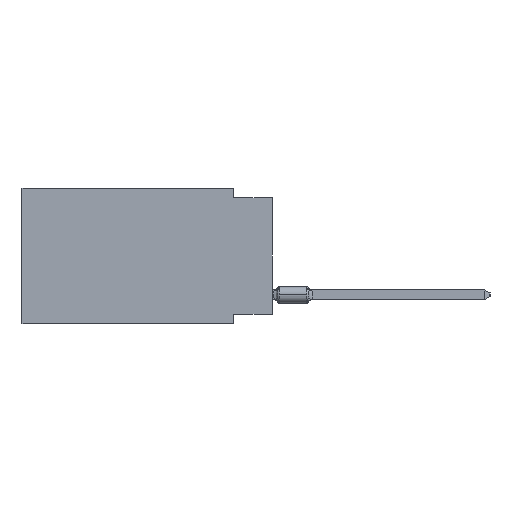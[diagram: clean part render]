
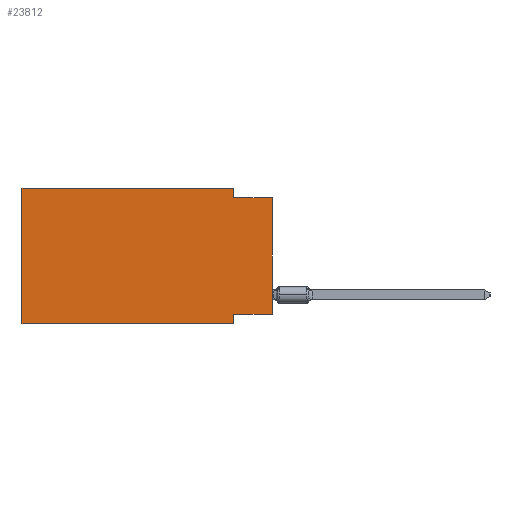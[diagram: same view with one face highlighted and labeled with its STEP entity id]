
A CAD part, left-side view. The second image highlights one B-rep face of the part: STEP entity #23812.
In plain terms, the highlighted planar face has unit normal (-1, 0, 0).
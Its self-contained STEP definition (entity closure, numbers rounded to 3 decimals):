
#1751 = CARTESIAN_POINT ( 'NONE',  ( 0., 16.383, 0. ) ) ;
#1979 = VERTEX_POINT ( 'NONE', #32588 ) ;
#2219 = VERTEX_POINT ( 'NONE', #20458 ) ;
#3049 = ORIENTED_EDGE ( 'NONE', *, *, #23880, .F. ) ;
#3287 = CARTESIAN_POINT ( 'NONE',  ( 0., 2.54, 0. ) ) ;
#4162 = VECTOR ( 'NONE', #24662, 1000. ) ;
#4232 = ORIENTED_EDGE ( 'NONE', *, *, #13092, .F. ) ;
#4549 = DIRECTION ( 'NONE',  ( 0., -1., 0. ) ) ;
#5205 = ORIENTED_EDGE ( 'NONE', *, *, #45596, .T. ) ;
#5371 = DIRECTION ( 'NONE',  ( 0., 0., -1. ) ) ;
#5651 = CARTESIAN_POINT ( 'NONE',  ( 0., 2.54, -8.255 ) ) ;
#5739 = VECTOR ( 'NONE', #15914, 1000. ) ;
#6019 = LINE ( 'NONE', #27401, #27716 ) ;
#7181 = LINE ( 'NONE', #21592, #31111 ) ;
#8831 = DIRECTION ( 'NONE',  ( 1., 0., 0. ) ) ;
#8984 = LINE ( 'NONE', #44307, #38594 ) ;
#9225 = DIRECTION ( 'NONE',  ( 0., 0., -1. ) ) ;
#10169 = LINE ( 'NONE', #18066, #14288 ) ;
#11076 = AXIS2_PLACEMENT_3D ( 'NONE', #31139, #8831, #5371 ) ;
#11493 = EDGE_CURVE ( 'NONE', #1979, #34793, #6019, .T. ) ;
#11506 = VERTEX_POINT ( 'NONE', #17597 ) ;
#13092 = EDGE_CURVE ( 'NONE', #28676, #11506, #8984, .T. ) ;
#13249 = FACE_OUTER_BOUND ( 'NONE', #34064, .T. ) ;
#13803 = ORIENTED_EDGE ( 'NONE', *, *, #22751, .F. ) ;
#14096 = VERTEX_POINT ( 'NONE', #21735 ) ;
#14211 = EDGE_CURVE ( 'NONE', #34793, #38241, #38218, .T. ) ;
#14288 = VECTOR ( 'NONE', #35498, 1000. ) ;
#15914 = DIRECTION ( 'NONE',  ( 0., -1., 0. ) ) ;
#16389 = CARTESIAN_POINT ( 'NONE',  ( 0., 0., -8.255 ) ) ;
#17597 = CARTESIAN_POINT ( 'NONE',  ( 0., 2.54, -8.89 ) ) ;
#18066 = CARTESIAN_POINT ( 'NONE',  ( 0., 0., -8.255 ) ) ;
#18703 = VECTOR ( 'NONE', #4549, 1000. ) ;
#20458 = CARTESIAN_POINT ( 'NONE',  ( 0., 0., -0.635 ) ) ;
#20572 = CARTESIAN_POINT ( 'NONE',  ( 0., 2.54, 0. ) ) ;
#20793 = DIRECTION ( 'NONE',  ( 0., 0., 1. ) ) ;
#20913 = DIRECTION ( 'NONE',  ( 0., -1., 0. ) ) ;
#21592 = CARTESIAN_POINT ( 'NONE',  ( 0., 0., -0.635 ) ) ;
#21735 = CARTESIAN_POINT ( 'NONE',  ( 0., 2.54, -0.635 ) ) ;
#22751 = EDGE_CURVE ( 'NONE', #30930, #28676, #10169, .T. ) ;
#23812 = ADVANCED_FACE ( 'NONE', ( #13249 ), #26518, .F. ) ;
#23880 = EDGE_CURVE ( 'NONE', #14096, #2219, #7181, .T. ) ;
#24662 = DIRECTION ( 'NONE',  ( 0., 0., -1. ) ) ;
#24781 = CARTESIAN_POINT ( 'NONE',  ( 0., 16.383, -8.89 ) ) ;
#24890 = LINE ( 'NONE', #3287, #4162 ) ;
#26378 = VECTOR ( 'NONE', #20793, 1000. ) ;
#26518 = PLANE ( 'NONE',  #11076 ) ;
#27401 = CARTESIAN_POINT ( 'NONE',  ( 0., 16.383, 0. ) ) ;
#27716 = VECTOR ( 'NONE', #31103, 1000. ) ;
#27773 = CARTESIAN_POINT ( 'NONE',  ( 0., 0., 0. ) ) ;
#28676 = VERTEX_POINT ( 'NONE', #5651 ) ;
#29860 = EDGE_CURVE ( 'NONE', #38241, #14096, #24890, .T. ) ;
#30930 = VERTEX_POINT ( 'NONE', #16389 ) ;
#31103 = DIRECTION ( 'NONE',  ( 0., 0., 1. ) ) ;
#31111 = VECTOR ( 'NONE', #20913, 1000. ) ;
#31139 = CARTESIAN_POINT ( 'NONE',  ( 0., 16.383, 0. ) ) ;
#32588 = CARTESIAN_POINT ( 'NONE',  ( 0., 16.383, -8.89 ) ) ;
#33971 = CARTESIAN_POINT ( 'NONE',  ( 0., 16.383, 0. ) ) ;
#34064 = EDGE_LOOP ( 'NONE', ( #42547, #3049, #36163, #37403, #40482, #5205, #4232, #13803 ) ) ;
#34793 = VERTEX_POINT ( 'NONE', #33971 ) ;
#35498 = DIRECTION ( 'NONE',  ( 0., 1., 0. ) ) ;
#36163 = ORIENTED_EDGE ( 'NONE', *, *, #29860, .F. ) ;
#36391 = LINE ( 'NONE', #24781, #18703 ) ;
#37403 = ORIENTED_EDGE ( 'NONE', *, *, #14211, .F. ) ;
#37775 = LINE ( 'NONE', #27773, #26378 ) ;
#38218 = LINE ( 'NONE', #1751, #5739 ) ;
#38241 = VERTEX_POINT ( 'NONE', #20572 ) ;
#38594 = VECTOR ( 'NONE', #9225, 1000. ) ;
#39390 = EDGE_CURVE ( 'NONE', #30930, #2219, #37775, .T. ) ;
#40482 = ORIENTED_EDGE ( 'NONE', *, *, #11493, .F. ) ;
#42547 = ORIENTED_EDGE ( 'NONE', *, *, #39390, .T. ) ;
#44307 = CARTESIAN_POINT ( 'NONE',  ( 0., 2.54, -8.89 ) ) ;
#45596 = EDGE_CURVE ( 'NONE', #1979, #11506, #36391, .T. ) ;
